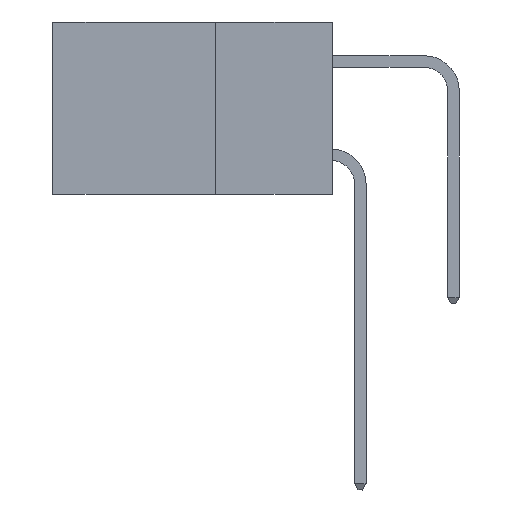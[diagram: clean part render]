
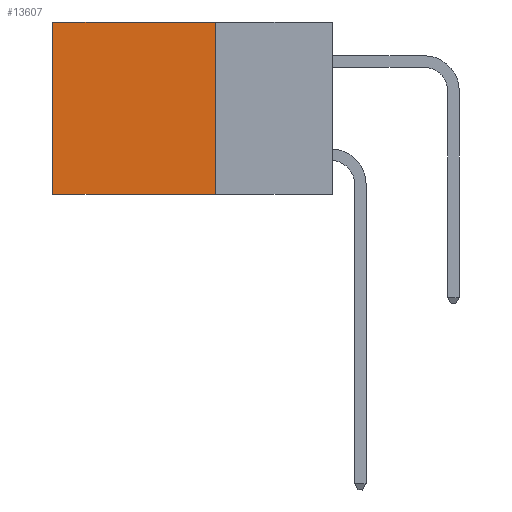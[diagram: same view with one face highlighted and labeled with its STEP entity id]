
A CAD part, left-side view. The second image highlights one B-rep face of the part: STEP entity #13607.
In plain terms, the highlighted planar face has unit normal (-1, 0, 0).
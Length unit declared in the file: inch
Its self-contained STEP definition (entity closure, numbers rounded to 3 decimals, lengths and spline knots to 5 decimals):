
#583 = VECTOR ( 'NONE', #12519, 39.37008 ) ;
#995 = CARTESIAN_POINT ( 'NONE',  ( 0.2615, 0.6, 0. ) ) ;
#1651 = ORIENTED_EDGE ( 'NONE', *, *, #12344, .F. ) ;
#1957 = PLANE ( 'NONE',  #3049 ) ;
#2352 = CARTESIAN_POINT ( 'NONE',  ( 0.2615, 0.6, -0.37 ) ) ;
#3049 = AXIS2_PLACEMENT_3D ( 'NONE', #14385, #11992, #3589 ) ;
#3171 = CARTESIAN_POINT ( 'NONE',  ( 0.2615, 0.25, -0.37 ) ) ;
#3589 = DIRECTION ( 'NONE',  ( 0., 0., -1. ) ) ;
#3626 = ORIENTED_EDGE ( 'NONE', *, *, #10179, .F. ) ;
#3940 = LINE ( 'NONE', #8321, #583 ) ;
#4727 = EDGE_LOOP ( 'NONE', ( #14194, #3626, #1651, #15104 ) ) ;
#6373 = VERTEX_POINT ( 'NONE', #995 ) ;
#7535 = VECTOR ( 'NONE', #8946, 39.37008 ) ;
#7934 = DIRECTION ( 'NONE',  ( 0., 0., -1. ) ) ;
#8321 = CARTESIAN_POINT ( 'NONE',  ( 0.2615, 0.25, 0. ) ) ;
#8706 = VECTOR ( 'NONE', #7934, 39.37008 ) ;
#8946 = DIRECTION ( 'NONE',  ( 0., 1., 0. ) ) ;
#9314 = LINE ( 'NONE', #2352, #8706 ) ;
#9581 = EDGE_CURVE ( 'NONE', #6373, #10308, #9314, .T. ) ;
#10179 = EDGE_CURVE ( 'NONE', #11490, #10308, #13139, .T. ) ;
#10308 = VERTEX_POINT ( 'NONE', #12407 ) ;
#10609 = CARTESIAN_POINT ( 'NONE',  ( 0.2615, 0.25, -0.37 ) ) ;
#10788 = EDGE_CURVE ( 'NONE', #16581, #6373, #3940, .T. ) ;
#11490 = VERTEX_POINT ( 'NONE', #10609 ) ;
#11691 = LINE ( 'NONE', #13598, #14740 ) ;
#11725 = FACE_OUTER_BOUND ( 'NONE', #4727, .T. ) ;
#11992 = DIRECTION ( 'NONE',  ( 1., 0., 0. ) ) ;
#12344 = EDGE_CURVE ( 'NONE', #16581, #11490, #11691, .T. ) ;
#12407 = CARTESIAN_POINT ( 'NONE',  ( 0.2615, 0.6, -0.37 ) ) ;
#12519 = DIRECTION ( 'NONE',  ( 0., 1., 0. ) ) ;
#13139 = LINE ( 'NONE', #3171, #7535 ) ;
#13598 = CARTESIAN_POINT ( 'NONE',  ( 0.2615, 0.25, -0.37 ) ) ;
#13607 = ADVANCED_FACE ( 'NONE', ( #11725 ), #1957, .F. ) ;
#14194 = ORIENTED_EDGE ( 'NONE', *, *, #9581, .T. ) ;
#14337 = DIRECTION ( 'NONE',  ( 0., 0., -1. ) ) ;
#14385 = CARTESIAN_POINT ( 'NONE',  ( 0.2615, 0.25, -0.37 ) ) ;
#14740 = VECTOR ( 'NONE', #14337, 39.37008 ) ;
#15104 = ORIENTED_EDGE ( 'NONE', *, *, #10788, .T. ) ;
#16170 = CARTESIAN_POINT ( 'NONE',  ( 0.2615, 0.25, 0. ) ) ;
#16581 = VERTEX_POINT ( 'NONE', #16170 ) ;
